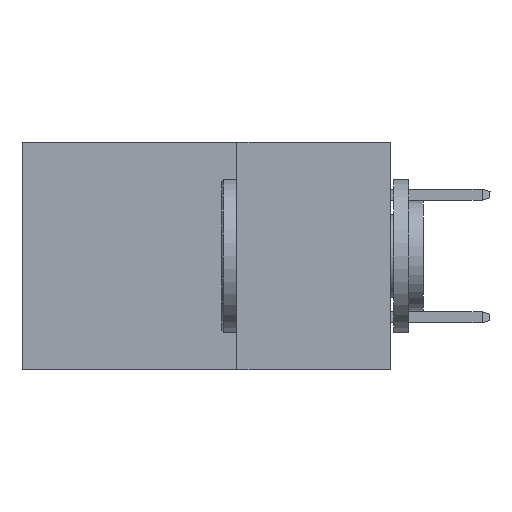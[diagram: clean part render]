
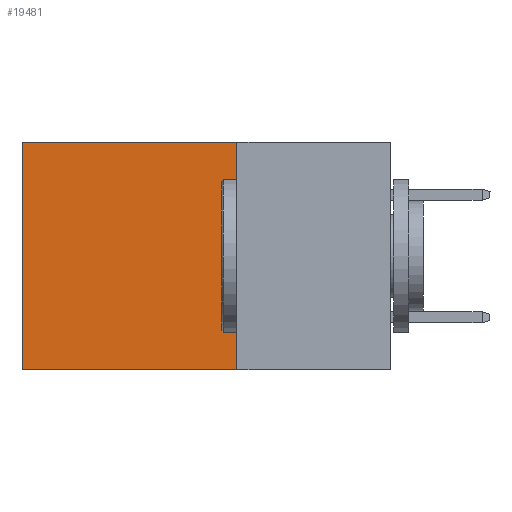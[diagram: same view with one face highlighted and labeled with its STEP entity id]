
A CAD part, left-side view. The second image highlights one B-rep face of the part: STEP entity #19481.
In plain terms, the highlighted planar face has unit normal (-1, 0, 0).
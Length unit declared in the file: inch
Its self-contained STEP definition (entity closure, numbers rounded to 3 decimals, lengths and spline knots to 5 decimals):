
#1347 = VECTOR ( 'NONE', #11998, 39.37008 ) ;
#1843 = AXIS2_PLACEMENT_3D ( 'NONE', #10215, #7182, #17980 ) ;
#2472 = ORIENTED_EDGE ( 'NONE', *, *, #3573, .F. ) ;
#2695 = FACE_OUTER_BOUND ( 'NONE', #9536, .T. ) ;
#2728 = CARTESIAN_POINT ( 'NONE',  ( 0.2875, 0.6, 0. ) ) ;
#3573 = EDGE_CURVE ( 'NONE', #18787, #10735, #19653, .T. ) ;
#4067 = CARTESIAN_POINT ( 'NONE',  ( 0.2875, 0.6, 0. ) ) ;
#5039 = VERTEX_POINT ( 'NONE', #4067 ) ;
#5332 = EDGE_CURVE ( 'NONE', #10735, #15803, #16691, .T. ) ;
#5595 = PLANE ( 'NONE',  #1843 ) ;
#6708 = LINE ( 'NONE', #7669, #10809 ) ;
#7182 = DIRECTION ( 'NONE',  ( 1., 0., 0. ) ) ;
#7338 = VECTOR ( 'NONE', #15896, 39.37008 ) ;
#7669 = CARTESIAN_POINT ( 'NONE',  ( 0.2875, 0.25, 0. ) ) ;
#8188 = CARTESIAN_POINT ( 'NONE',  ( 0.2875, 0.25, 0. ) ) ;
#8539 = ORIENTED_EDGE ( 'NONE', *, *, #10439, .T. ) ;
#9411 = CARTESIAN_POINT ( 'NONE',  ( 0.2875, 0.25, -0.37 ) ) ;
#9536 = EDGE_LOOP ( 'NONE', ( #20021, #16623, #2472, #8539 ) ) ;
#10215 = CARTESIAN_POINT ( 'NONE',  ( 0.2875, 0.25, 0. ) ) ;
#10322 = EDGE_CURVE ( 'NONE', #5039, #15803, #17349, .T. ) ;
#10439 = EDGE_CURVE ( 'NONE', #18787, #5039, #6708, .T. ) ;
#10735 = VERTEX_POINT ( 'NONE', #11381 ) ;
#10809 = VECTOR ( 'NONE', #18481, 39.37008 ) ;
#11381 = CARTESIAN_POINT ( 'NONE',  ( 0.2875, 0.25, -0.37 ) ) ;
#11998 = DIRECTION ( 'NONE',  ( 0., 0., -1. ) ) ;
#12534 = VECTOR ( 'NONE', #15635, 39.37008 ) ;
#13111 = CARTESIAN_POINT ( 'NONE',  ( 0.2875, 0.25, 0. ) ) ;
#15635 = DIRECTION ( 'NONE',  ( 0., 1., 0. ) ) ;
#15803 = VERTEX_POINT ( 'NONE', #19029 ) ;
#15896 = DIRECTION ( 'NONE',  ( 0., 0., -1. ) ) ;
#16623 = ORIENTED_EDGE ( 'NONE', *, *, #5332, .F. ) ;
#16691 = LINE ( 'NONE', #9411, #12534 ) ;
#17349 = LINE ( 'NONE', #2728, #1347 ) ;
#17980 = DIRECTION ( 'NONE',  ( 0., 0., -1. ) ) ;
#18481 = DIRECTION ( 'NONE',  ( 0., 1., 0. ) ) ;
#18787 = VERTEX_POINT ( 'NONE', #13111 ) ;
#19029 = CARTESIAN_POINT ( 'NONE',  ( 0.2875, 0.6, -0.37 ) ) ;
#19481 = ADVANCED_FACE ( 'NONE', ( #2695 ), #5595, .F. ) ;
#19653 = LINE ( 'NONE', #8188, #7338 ) ;
#20021 = ORIENTED_EDGE ( 'NONE', *, *, #10322, .T. ) ;
